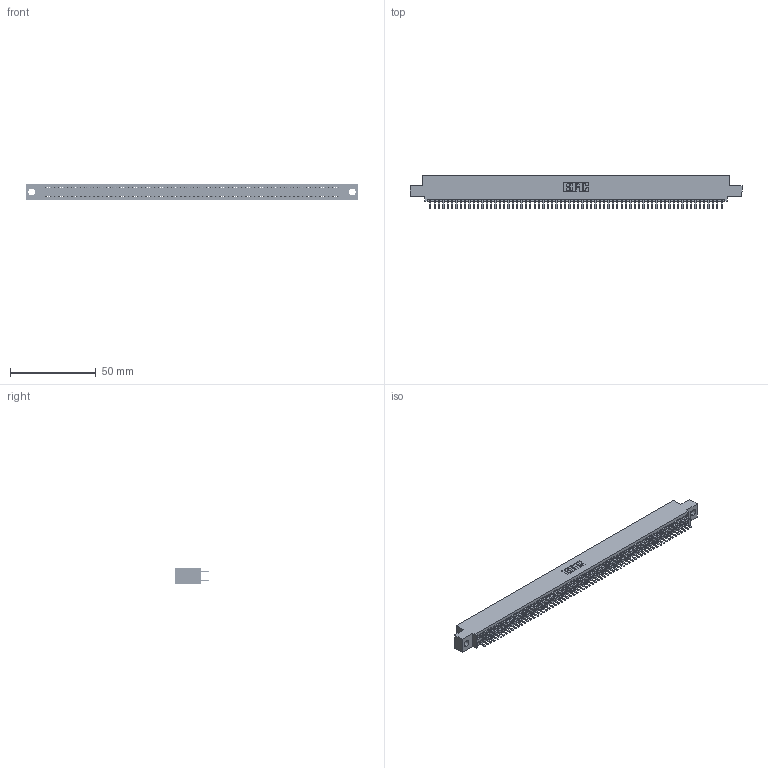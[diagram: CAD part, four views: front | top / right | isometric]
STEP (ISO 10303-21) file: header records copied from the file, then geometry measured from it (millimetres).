
FILE_DESCRIPTION (( 'STEP AP203' ), '1' );
FILE_NAME ('395-136-520-504.STEP', '2021-06-18T02:26:32', ( '' ), ( '' ), 'SwSTEP 2.0', 'SolidWorks 2020', '' );
FILE_SCHEMA (( 'CONFIG_CONTROL_DESIGN' ));
Length unit declared in the file: inch
Products named in the file (3): 395-136-520-504; 345 Part_0.110 Offset - 0.156 Dia-TI; 345-292-001_345-293-120
Assembly tree (137 placements, depth 2):
  395-136-520-504
    345 Part_0.110 Offset - 0.156 Dia-TI
    345-292-001_345-293-120  x136
Bounding box: 193.93 x 19.68 x 9.4 mm (x, y, z)
Volume: 18840.7 mm3; surface area: 28170.5 mm2
Topology: 137 solids, 137 shells, 7488 faces, 21741 edges, 14130 vertices
Faces by surface type: plane 4858, cylinder 2630
Entity records: 50519 total; most frequent: CARTESIAN_POINT 8462, ORIENTED_EDGE 8382, DIRECTION 7415, EDGE_CURVE 4191, LINE 3783, VECTOR 3783, VERTEX_POINT 2790, AXIS2_PLACEMENT_3D 1816
